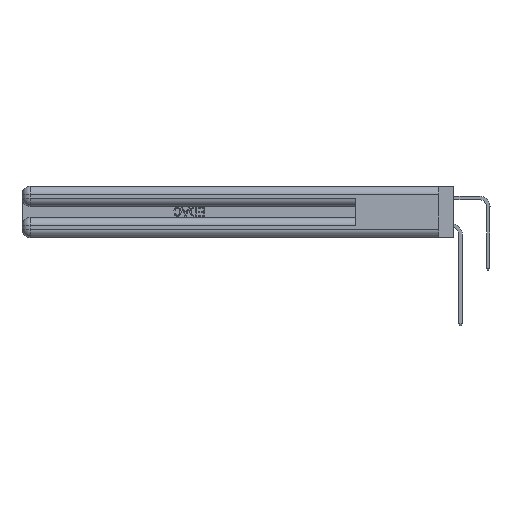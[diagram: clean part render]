
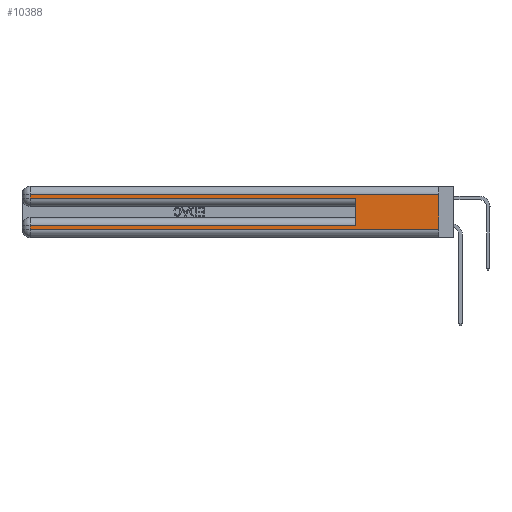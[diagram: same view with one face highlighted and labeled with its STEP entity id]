
A CAD part, left-side view. The second image highlights one B-rep face of the part: STEP entity #10388.
In plain terms, the highlighted planar face has unit normal (-1, 0, 0).
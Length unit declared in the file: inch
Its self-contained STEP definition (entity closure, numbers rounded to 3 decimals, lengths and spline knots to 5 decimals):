
#133 = VERTEX_POINT ( 'NONE', #31119 ) ;
#1327 = EDGE_CURVE ( 'NONE', #3012, #26501, #7520, .T. ) ;
#3012 = VERTEX_POINT ( 'NONE', #34722 ) ;
#3283 = VECTOR ( 'NONE', #9390, 39.37008 ) ;
#3437 = VERTEX_POINT ( 'NONE', #36983 ) ;
#4909 = ORIENTED_EDGE ( 'NONE', *, *, #40355, .T. ) ;
#5154 = ORIENTED_EDGE ( 'NONE', *, *, #9174, .T. ) ;
#5175 = LINE ( 'NONE', #7198, #35556 ) ;
#5554 = CARTESIAN_POINT ( 'NONE',  ( 0., 0., 0.085 ) ) ;
#5783 = LINE ( 'NONE', #15304, #6739 ) ;
#6391 = AXIS2_PLACEMENT_3D ( 'NONE', #26299, #36681, #23648 ) ;
#6739 = VECTOR ( 'NONE', #40563, 39.37008 ) ;
#7198 = CARTESIAN_POINT ( 'NONE',  ( 0., 2.94, 0.37 ) ) ;
#7458 = PLANE ( 'NONE',  #6391 ) ;
#7520 = LINE ( 'NONE', #31187, #16326 ) ;
#7569 = VERTEX_POINT ( 'NONE', #26245 ) ;
#9015 = CARTESIAN_POINT ( 'NONE',  ( 0., 0.6, 0.285 ) ) ;
#9055 = EDGE_LOOP ( 'NONE', ( #17160, #39459, #21195, #38341, #39753, #5154, #33338, #4909 ) ) ;
#9174 = EDGE_CURVE ( 'NONE', #24200, #7569, #34063, .T. ) ;
#9390 = DIRECTION ( 'NONE',  ( 0., 0., -1. ) ) ;
#9544 = LINE ( 'NONE', #15145, #10001 ) ;
#10001 = VECTOR ( 'NONE', #15431, 39.37008 ) ;
#10388 = ADVANCED_FACE ( 'NONE', ( #39821 ), #7458, .F. ) ;
#11066 = LINE ( 'NONE', #12427, #3283 ) ;
#12284 = VERTEX_POINT ( 'NONE', #21397 ) ;
#12418 = DIRECTION ( 'NONE',  ( 0., -1., 0. ) ) ;
#12427 = CARTESIAN_POINT ( 'NONE',  ( 0., 0., 0.37 ) ) ;
#15145 = CARTESIAN_POINT ( 'NONE',  ( 0., 0.6, 0.145 ) ) ;
#15304 = CARTESIAN_POINT ( 'NONE',  ( 0., 0., 0.31 ) ) ;
#15431 = DIRECTION ( 'NONE',  ( 0., 0., 1. ) ) ;
#16326 = VECTOR ( 'NONE', #12418, 39.37008 ) ;
#17160 = ORIENTED_EDGE ( 'NONE', *, *, #18873, .F. ) ;
#18873 = EDGE_CURVE ( 'NONE', #133, #28451, #11066, .T. ) ;
#19308 = EDGE_CURVE ( 'NONE', #24200, #26501, #9544, .T. ) ;
#19624 = VECTOR ( 'NONE', #29728, 39.37008 ) ;
#19856 = EDGE_CURVE ( 'NONE', #12284, #3012, #5175, .T. ) ;
#21152 = EDGE_CURVE ( 'NONE', #133, #12284, #5783, .T. ) ;
#21195 = ORIENTED_EDGE ( 'NONE', *, *, #19856, .T. ) ;
#21397 = CARTESIAN_POINT ( 'NONE',  ( 0., 2.94, 0.31 ) ) ;
#22950 = CARTESIAN_POINT ( 'NONE',  ( 0., 0., 0.06 ) ) ;
#23648 = DIRECTION ( 'NONE',  ( 0., 0., -1. ) ) ;
#24200 = VERTEX_POINT ( 'NONE', #31667 ) ;
#24282 = CARTESIAN_POINT ( 'NONE',  ( 0., 0., 0.06 ) ) ;
#25494 = DIRECTION ( 'NONE',  ( 0., 0., -1. ) ) ;
#26245 = CARTESIAN_POINT ( 'NONE',  ( 0., 2.94, 0.085 ) ) ;
#26299 = CARTESIAN_POINT ( 'NONE',  ( 0., 0., 0.37 ) ) ;
#26501 = VERTEX_POINT ( 'NONE', #9015 ) ;
#26618 = VECTOR ( 'NONE', #29578, 39.37008 ) ;
#27102 = LINE ( 'NONE', #39089, #26618 ) ;
#27374 = DIRECTION ( 'NONE',  ( 0., 1., 0. ) ) ;
#28451 = VERTEX_POINT ( 'NONE', #24282 ) ;
#29578 = DIRECTION ( 'NONE',  ( 0., 0., -1. ) ) ;
#29728 = DIRECTION ( 'NONE',  ( 0., -1., 0. ) ) ;
#31119 = CARTESIAN_POINT ( 'NONE',  ( 0., 0., 0.31 ) ) ;
#31187 = CARTESIAN_POINT ( 'NONE',  ( 0., 0., 0.285 ) ) ;
#31468 = LINE ( 'NONE', #22950, #19624 ) ;
#31667 = CARTESIAN_POINT ( 'NONE',  ( 0., 0.6, 0.085 ) ) ;
#33054 = VECTOR ( 'NONE', #27374, 39.37008 ) ;
#33338 = ORIENTED_EDGE ( 'NONE', *, *, #39308, .T. ) ;
#34063 = LINE ( 'NONE', #5554, #33054 ) ;
#34722 = CARTESIAN_POINT ( 'NONE',  ( 0., 2.94, 0.285 ) ) ;
#35556 = VECTOR ( 'NONE', #25494, 39.37008 ) ;
#36681 = DIRECTION ( 'NONE',  ( 1., 0., 0. ) ) ;
#36983 = CARTESIAN_POINT ( 'NONE',  ( 0., 2.94, 0.06 ) ) ;
#38341 = ORIENTED_EDGE ( 'NONE', *, *, #1327, .T. ) ;
#39089 = CARTESIAN_POINT ( 'NONE',  ( 0., 2.94, 0.37 ) ) ;
#39308 = EDGE_CURVE ( 'NONE', #7569, #3437, #27102, .T. ) ;
#39459 = ORIENTED_EDGE ( 'NONE', *, *, #21152, .T. ) ;
#39753 = ORIENTED_EDGE ( 'NONE', *, *, #19308, .F. ) ;
#39821 = FACE_OUTER_BOUND ( 'NONE', #9055, .T. ) ;
#40355 = EDGE_CURVE ( 'NONE', #3437, #28451, #31468, .T. ) ;
#40563 = DIRECTION ( 'NONE',  ( 0., 1., 0. ) ) ;
